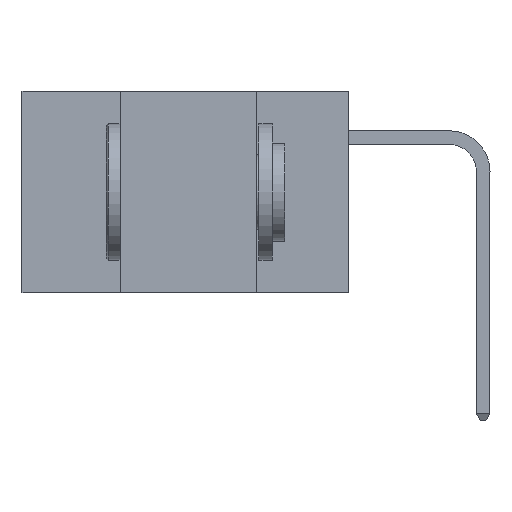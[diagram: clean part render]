
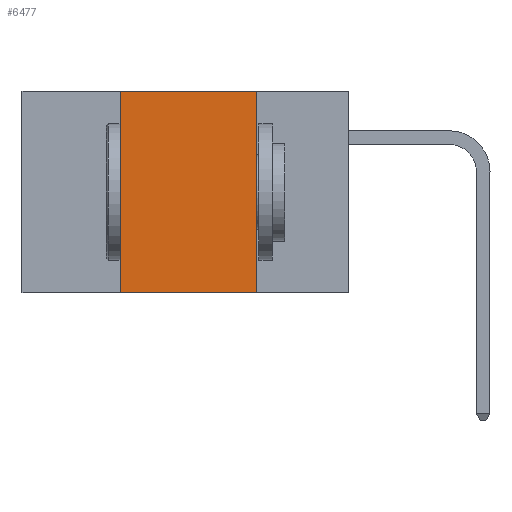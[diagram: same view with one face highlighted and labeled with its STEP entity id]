
A CAD part, left-side view. The second image highlights one B-rep face of the part: STEP entity #6477.
In plain terms, the highlighted planar face has unit normal (-1, 0, 0).
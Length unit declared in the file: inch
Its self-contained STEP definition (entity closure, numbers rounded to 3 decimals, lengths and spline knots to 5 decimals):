
#13 = LINE ( 'NONE', #12875, #3327 ) ;
#663 = CARTESIAN_POINT ( 'NONE',  ( 0., 0.6, 0. ) ) ;
#2301 = FACE_OUTER_BOUND ( 'NONE', #10679, .T. ) ;
#2945 = VERTEX_POINT ( 'NONE', #28779 ) ;
#2975 = EDGE_CURVE ( 'NONE', #29475, #2945, #32044, .T. ) ;
#3327 = VECTOR ( 'NONE', #15217, 39.37008 ) ;
#4611 = VECTOR ( 'NONE', #34330, 39.37008 ) ;
#4617 = ORIENTED_EDGE ( 'NONE', *, *, #28125, .F. ) ;
#6093 = VERTEX_POINT ( 'NONE', #24361 ) ;
#6477 = ADVANCED_FACE ( 'NONE', ( #2301 ), #16163, .F. ) ;
#7187 = DIRECTION ( 'NONE',  ( 1., 0., 0. ) ) ;
#7489 = LINE ( 'NONE', #21115, #4611 ) ;
#10679 = EDGE_LOOP ( 'NONE', ( #31295, #24893, #4617, #10824 ) ) ;
#10824 = ORIENTED_EDGE ( 'NONE', *, *, #27351, .T. ) ;
#10831 = VECTOR ( 'NONE', #16196, 39.37008 ) ;
#11747 = DIRECTION ( 'NONE',  ( 0., 0., -1. ) ) ;
#12875 = CARTESIAN_POINT ( 'NONE',  ( 0., 0.42, 0. ) ) ;
#13523 = DIRECTION ( 'NONE',  ( 0., 0., -1. ) ) ;
#15217 = DIRECTION ( 'NONE',  ( 0., 0., 1. ) ) ;
#16163 = PLANE ( 'NONE',  #18886 ) ;
#16196 = DIRECTION ( 'NONE',  ( 0., -1., 0. ) ) ;
#16994 = CARTESIAN_POINT ( 'NONE',  ( 0., 0.17, 0. ) ) ;
#18886 = AXIS2_PLACEMENT_3D ( 'NONE', #663, #7187, #13523 ) ;
#20115 = VERTEX_POINT ( 'NONE', #21318 ) ;
#21115 = CARTESIAN_POINT ( 'NONE',  ( 0., 0.6, -0.37 ) ) ;
#21278 = VECTOR ( 'NONE', #11747, 39.37008 ) ;
#21318 = CARTESIAN_POINT ( 'NONE',  ( 0., 0.42, -0.37 ) ) ;
#23861 = CARTESIAN_POINT ( 'NONE',  ( 0., 0.42, 0. ) ) ;
#24361 = CARTESIAN_POINT ( 'NONE',  ( 0., 0.17, -0.37 ) ) ;
#24893 = ORIENTED_EDGE ( 'NONE', *, *, #2975, .F. ) ;
#26539 = EDGE_CURVE ( 'NONE', #2945, #6093, #29589, .T. ) ;
#27351 = EDGE_CURVE ( 'NONE', #20115, #6093, #7489, .T. ) ;
#28125 = EDGE_CURVE ( 'NONE', #20115, #29475, #13, .T. ) ;
#28779 = CARTESIAN_POINT ( 'NONE',  ( 0., 0.17, 0. ) ) ;
#29472 = CARTESIAN_POINT ( 'NONE',  ( 0., 0.6, 0. ) ) ;
#29475 = VERTEX_POINT ( 'NONE', #23861 ) ;
#29589 = LINE ( 'NONE', #16994, #21278 ) ;
#31295 = ORIENTED_EDGE ( 'NONE', *, *, #26539, .F. ) ;
#32044 = LINE ( 'NONE', #29472, #10831 ) ;
#34330 = DIRECTION ( 'NONE',  ( 0., -1., 0. ) ) ;
